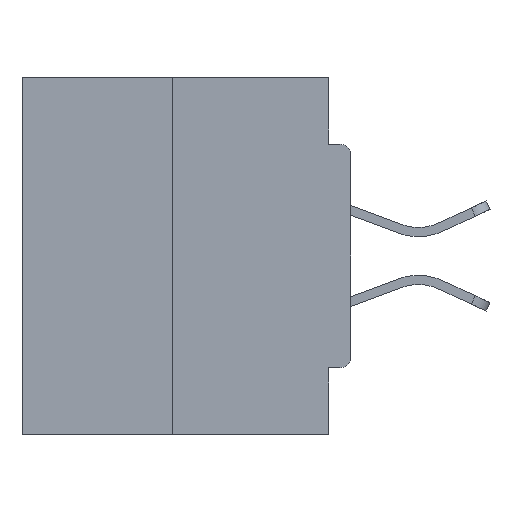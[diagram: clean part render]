
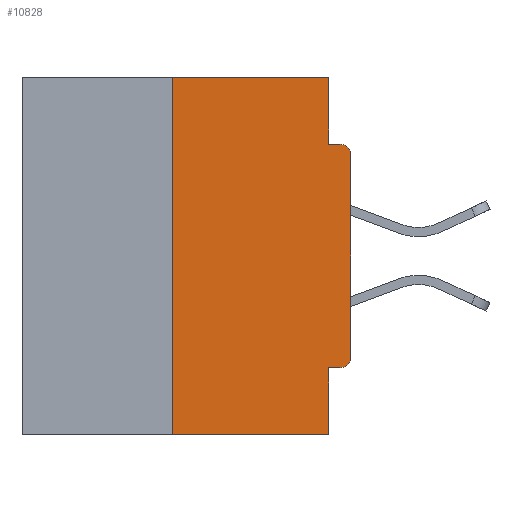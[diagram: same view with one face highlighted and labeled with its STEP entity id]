
A CAD part, left-side view. The second image highlights one B-rep face of the part: STEP entity #10828.
In plain terms, the highlighted planar face has unit normal (-1, 0, 0).
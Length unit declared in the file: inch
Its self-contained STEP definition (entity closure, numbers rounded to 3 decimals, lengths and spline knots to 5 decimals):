
#78 = CARTESIAN_POINT ( 'NONE',  ( 0., 0., -0.4065 ) ) ;
#763 = AXIS2_PLACEMENT_3D ( 'NONE', #16443, #29095, #11172 ) ;
#1517 = CARTESIAN_POINT ( 'NONE',  ( 0., 0.25, 0. ) ) ;
#1642 = ORIENTED_EDGE ( 'NONE', *, *, #18387, .F. ) ;
#1753 = AXIS2_PLACEMENT_3D ( 'NONE', #6478, #32191, #3876 ) ;
#1885 = VERTEX_POINT ( 'NONE', #26715 ) ;
#2420 = VERTEX_POINT ( 'NONE', #5437 ) ;
#2805 = ORIENTED_EDGE ( 'NONE', *, *, #26028, .T. ) ;
#2892 = CARTESIAN_POINT ( 'NONE',  ( 0., 0.25, 0. ) ) ;
#2975 = VECTOR ( 'NONE', #3595, 39.37008 ) ;
#3097 = CARTESIAN_POINT ( 'NONE',  ( 0., 0.031, -0.0935 ) ) ;
#3326 = DIRECTION ( 'NONE',  ( 0., 0., 1. ) ) ;
#3549 = CARTESIAN_POINT ( 'NONE',  ( 0., 0.46, 0. ) ) ;
#3595 = DIRECTION ( 'NONE',  ( 0., -1., 0. ) ) ;
#3710 = VECTOR ( 'NONE', #7787, 39.37008 ) ;
#3785 = DIRECTION ( 'NONE',  ( 0., 0., -1. ) ) ;
#3876 = DIRECTION ( 'NONE',  ( 0., 0., -1. ) ) ;
#4198 = EDGE_LOOP ( 'NONE', ( #23699, #22591, #5234, #1642, #30037, #2805, #19136, #26735, #24241, #29574 ) ) ;
#4619 = EDGE_CURVE ( 'NONE', #2420, #6845, #5282, .T. ) ;
#4741 = FACE_OUTER_BOUND ( 'NONE', #4198, .T. ) ;
#5234 = ORIENTED_EDGE ( 'NONE', *, *, #30987, .T. ) ;
#5282 = LINE ( 'NONE', #20888, #18206 ) ;
#5437 = CARTESIAN_POINT ( 'NONE',  ( 0., 0.031, 0. ) ) ;
#6478 = CARTESIAN_POINT ( 'NONE',  ( 0., 0.015, -0.3915 ) ) ;
#6666 = CARTESIAN_POINT ( 'NONE',  ( 0., 0., 0. ) ) ;
#6845 = VERTEX_POINT ( 'NONE', #3097 ) ;
#6944 = LINE ( 'NONE', #6666, #3710 ) ;
#7787 = DIRECTION ( 'NONE',  ( 0., 0., 1. ) ) ;
#8126 = DIRECTION ( 'NONE',  ( 0., 0., -1. ) ) ;
#9306 = VECTOR ( 'NONE', #13586, 39.37008 ) ;
#9947 = VECTOR ( 'NONE', #29259, 39.37008 ) ;
#10828 = ADVANCED_FACE ( 'NONE', ( #4741 ), #13835, .F. ) ;
#11021 = VERTEX_POINT ( 'NONE', #22183 ) ;
#11046 = CIRCLE ( 'NONE', #763, 0.015 ) ;
#11172 = DIRECTION ( 'NONE',  ( 0., 0., -1. ) ) ;
#13586 = DIRECTION ( 'NONE',  ( 0., 1., 0. ) ) ;
#13835 = PLANE ( 'NONE',  #20393 ) ;
#14466 = EDGE_CURVE ( 'NONE', #16870, #2420, #20445, .T. ) ;
#15204 = EDGE_CURVE ( 'NONE', #6845, #17315, #21625, .T. ) ;
#16345 = VECTOR ( 'NONE', #29546, 39.37008 ) ;
#16443 = CARTESIAN_POINT ( 'NONE',  ( 0., 0.015, -0.1085 ) ) ;
#16639 = DIRECTION ( 'NONE',  ( 1., 0., 0. ) ) ;
#16870 = VERTEX_POINT ( 'NONE', #2892 ) ;
#16914 = CARTESIAN_POINT ( 'NONE',  ( 0., 0.015, -0.4065 ) ) ;
#17136 = CARTESIAN_POINT ( 'NONE',  ( 0., 0.015, -0.0935 ) ) ;
#17315 = VERTEX_POINT ( 'NONE', #17136 ) ;
#17363 = CARTESIAN_POINT ( 'NONE',  ( 0., 0.25, -0.5 ) ) ;
#17424 = VERTEX_POINT ( 'NONE', #17524 ) ;
#17524 = CARTESIAN_POINT ( 'NONE',  ( 0., 0.031, -0.5 ) ) ;
#17569 = EDGE_CURVE ( 'NONE', #26297, #1885, #6944, .T. ) ;
#18206 = VECTOR ( 'NONE', #8126, 39.37008 ) ;
#18228 = VECTOR ( 'NONE', #33286, 39.37008 ) ;
#18387 = EDGE_CURVE ( 'NONE', #11021, #17424, #23089, .T. ) ;
#18410 = CARTESIAN_POINT ( 'NONE',  ( 0., 0., -0.3915 ) ) ;
#18599 = VECTOR ( 'NONE', #3326, 39.37008 ) ;
#19136 = ORIENTED_EDGE ( 'NONE', *, *, #17569, .T. ) ;
#19402 = LINE ( 'NONE', #1517, #18599 ) ;
#20393 = AXIS2_PLACEMENT_3D ( 'NONE', #3549, #16639, #3785 ) ;
#20445 = LINE ( 'NONE', #29495, #9947 ) ;
#20620 = LINE ( 'NONE', #78, #9306 ) ;
#20888 = CARTESIAN_POINT ( 'NONE',  ( 0., 0.031, 0. ) ) ;
#21292 = VERTEX_POINT ( 'NONE', #17363 ) ;
#21625 = LINE ( 'NONE', #29763, #16345 ) ;
#22183 = CARTESIAN_POINT ( 'NONE',  ( 0., 0.031, -0.4065 ) ) ;
#22364 = LINE ( 'NONE', #22370, #2975 ) ;
#22370 = CARTESIAN_POINT ( 'NONE',  ( 0., 0.46, -0.5 ) ) ;
#22591 = ORIENTED_EDGE ( 'NONE', *, *, #26491, .F. ) ;
#23089 = LINE ( 'NONE', #30691, #18228 ) ;
#23699 = ORIENTED_EDGE ( 'NONE', *, *, #14466, .F. ) ;
#24241 = ORIENTED_EDGE ( 'NONE', *, *, #15204, .F. ) ;
#25909 = CIRCLE ( 'NONE', #1753, 0.015 ) ;
#26028 = EDGE_CURVE ( 'NONE', #33135, #26297, #25909, .T. ) ;
#26297 = VERTEX_POINT ( 'NONE', #18410 ) ;
#26491 = EDGE_CURVE ( 'NONE', #21292, #16870, #19402, .T. ) ;
#26496 = EDGE_CURVE ( 'NONE', #33135, #11021, #20620, .T. ) ;
#26715 = CARTESIAN_POINT ( 'NONE',  ( 0., 0., -0.1085 ) ) ;
#26735 = ORIENTED_EDGE ( 'NONE', *, *, #31084, .T. ) ;
#29095 = DIRECTION ( 'NONE',  ( -1., 0., 0. ) ) ;
#29259 = DIRECTION ( 'NONE',  ( 0., -1., 0. ) ) ;
#29495 = CARTESIAN_POINT ( 'NONE',  ( 0., 0.46, 0. ) ) ;
#29546 = DIRECTION ( 'NONE',  ( 0., -1., 0. ) ) ;
#29574 = ORIENTED_EDGE ( 'NONE', *, *, #4619, .F. ) ;
#29763 = CARTESIAN_POINT ( 'NONE',  ( 0., 0., -0.0935 ) ) ;
#30037 = ORIENTED_EDGE ( 'NONE', *, *, #26496, .F. ) ;
#30691 = CARTESIAN_POINT ( 'NONE',  ( 0., 0.031, -0.5 ) ) ;
#30987 = EDGE_CURVE ( 'NONE', #21292, #17424, #22364, .T. ) ;
#31084 = EDGE_CURVE ( 'NONE', #1885, #17315, #11046, .T. ) ;
#32191 = DIRECTION ( 'NONE',  ( -1., 0., 0. ) ) ;
#33135 = VERTEX_POINT ( 'NONE', #16914 ) ;
#33286 = DIRECTION ( 'NONE',  ( 0., 0., -1. ) ) ;
